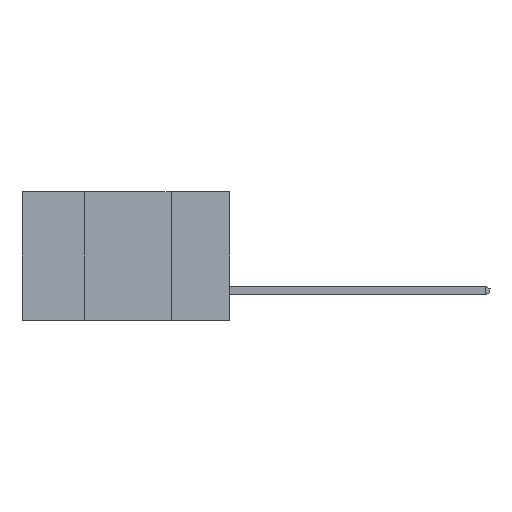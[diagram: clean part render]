
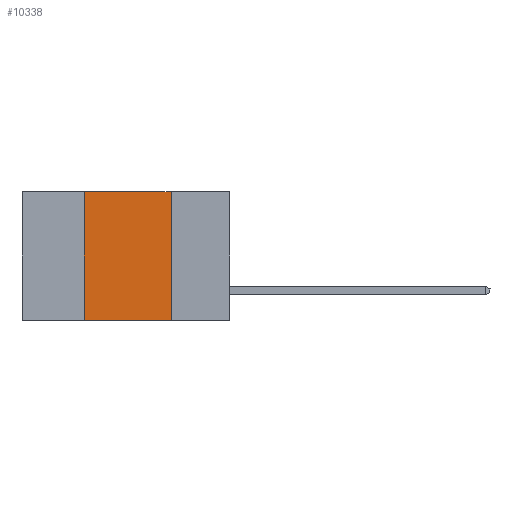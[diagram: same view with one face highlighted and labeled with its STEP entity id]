
A CAD part, left-side view. The second image highlights one B-rep face of the part: STEP entity #10338.
In plain terms, the highlighted planar face has unit normal (-1, 0, 0).
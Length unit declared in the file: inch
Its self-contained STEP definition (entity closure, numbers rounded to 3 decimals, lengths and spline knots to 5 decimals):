
#243 = DIRECTION ( 'NONE',  ( 0., -1., 0. ) ) ;
#879 = CARTESIAN_POINT ( 'NONE',  ( 0., 0.42, 0. ) ) ;
#1125 = DIRECTION ( 'NONE',  ( 0., -1., 0. ) ) ;
#1606 = CARTESIAN_POINT ( 'NONE',  ( 0., 0.17, 0. ) ) ;
#1740 = VECTOR ( 'NONE', #1125, 39.37008 ) ;
#1757 = VECTOR ( 'NONE', #7043, 39.37008 ) ;
#2389 = PLANE ( 'NONE',  #3846 ) ;
#2950 = VERTEX_POINT ( 'NONE', #10377 ) ;
#3200 = EDGE_CURVE ( 'NONE', #2950, #4615, #7245, .T. ) ;
#3398 = ORIENTED_EDGE ( 'NONE', *, *, #7080, .F. ) ;
#3846 = AXIS2_PLACEMENT_3D ( 'NONE', #8424, #11424, #6352 ) ;
#4313 = CARTESIAN_POINT ( 'NONE',  ( 0., 0.6, 0. ) ) ;
#4615 = VERTEX_POINT ( 'NONE', #8809 ) ;
#4891 = ORIENTED_EDGE ( 'NONE', *, *, #7598, .F. ) ;
#5112 = VERTEX_POINT ( 'NONE', #879 ) ;
#6086 = VECTOR ( 'NONE', #11632, 39.37008 ) ;
#6352 = DIRECTION ( 'NONE',  ( 0., 0., -1. ) ) ;
#6397 = ORIENTED_EDGE ( 'NONE', *, *, #3200, .T. ) ;
#6411 = FACE_OUTER_BOUND ( 'NONE', #9501, .T. ) ;
#6985 = CARTESIAN_POINT ( 'NONE',  ( 0., 0.42, -0.37 ) ) ;
#7043 = DIRECTION ( 'NONE',  ( 0., 0., 1. ) ) ;
#7080 = EDGE_CURVE ( 'NONE', #12185, #4615, #7664, .T. ) ;
#7245 = LINE ( 'NONE', #12004, #8513 ) ;
#7598 = EDGE_CURVE ( 'NONE', #5112, #12185, #11978, .T. ) ;
#7664 = LINE ( 'NONE', #10898, #6086 ) ;
#8424 = CARTESIAN_POINT ( 'NONE',  ( 0., 0.6, 0. ) ) ;
#8513 = VECTOR ( 'NONE', #243, 39.37008 ) ;
#8809 = CARTESIAN_POINT ( 'NONE',  ( 0., 0.17, -0.37 ) ) ;
#9501 = EDGE_LOOP ( 'NONE', ( #3398, #4891, #11143, #6397 ) ) ;
#9759 = EDGE_CURVE ( 'NONE', #2950, #5112, #9769, .T. ) ;
#9769 = LINE ( 'NONE', #6985, #1757 ) ;
#10338 = ADVANCED_FACE ( 'NONE', ( #6411 ), #2389, .F. ) ;
#10377 = CARTESIAN_POINT ( 'NONE',  ( 0., 0.42, -0.37 ) ) ;
#10898 = CARTESIAN_POINT ( 'NONE',  ( 0., 0.17, -0.37 ) ) ;
#11143 = ORIENTED_EDGE ( 'NONE', *, *, #9759, .F. ) ;
#11424 = DIRECTION ( 'NONE',  ( 1., 0., 0. ) ) ;
#11632 = DIRECTION ( 'NONE',  ( 0., 0., -1. ) ) ;
#11978 = LINE ( 'NONE', #4313, #1740 ) ;
#12004 = CARTESIAN_POINT ( 'NONE',  ( 0., 0.6, -0.37 ) ) ;
#12185 = VERTEX_POINT ( 'NONE', #1606 ) ;
